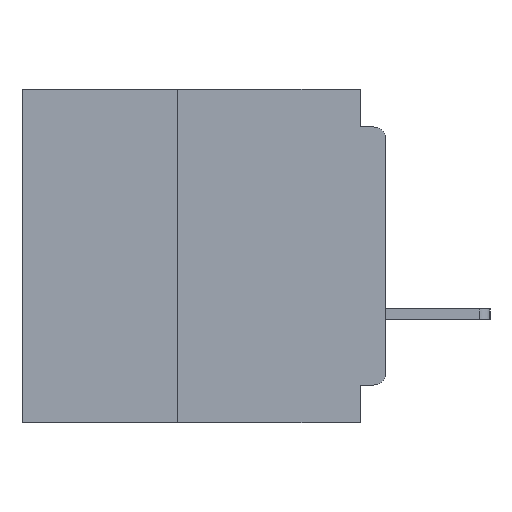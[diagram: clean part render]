
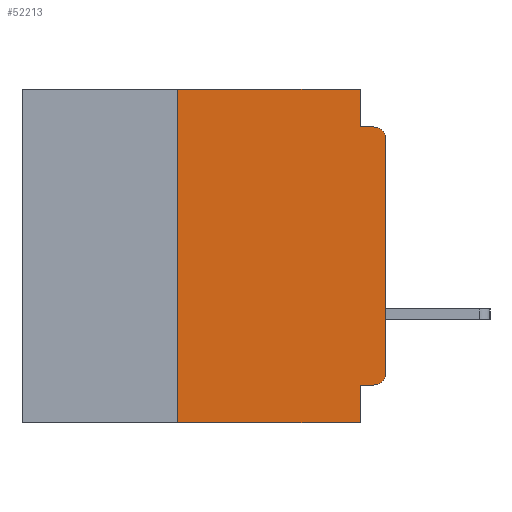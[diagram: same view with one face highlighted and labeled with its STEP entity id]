
A CAD part, left-side view. The second image highlights one B-rep face of the part: STEP entity #52213.
In plain terms, the highlighted planar face has unit normal (-1, 0, 0).
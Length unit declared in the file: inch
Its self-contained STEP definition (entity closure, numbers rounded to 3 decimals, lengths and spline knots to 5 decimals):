
#1529 = CARTESIAN_POINT ( 'NONE',  ( 0., 0., 0. ) ) ;
#2550 = CARTESIAN_POINT ( 'NONE',  ( 0., 0.015, -0.34 ) ) ;
#2847 = CARTESIAN_POINT ( 'NONE',  ( 0., 0.031, 0. ) ) ;
#3229 = CARTESIAN_POINT ( 'NONE',  ( 0., 0.015, -0.355 ) ) ;
#4304 = CARTESIAN_POINT ( 'NONE',  ( 0., 0.437, 0. ) ) ;
#5494 = CARTESIAN_POINT ( 'NONE',  ( 0., 0.25, -0.4 ) ) ;
#7000 = CIRCLE ( 'NONE', #40093, 0.015 ) ;
#7048 = DIRECTION ( 'NONE',  ( 0., 0., -1. ) ) ;
#8974 = CARTESIAN_POINT ( 'NONE',  ( 0., 0.25, -0.4 ) ) ;
#9078 = CARTESIAN_POINT ( 'NONE',  ( 0., 0.031, -0.045 ) ) ;
#9638 = LINE ( 'NONE', #50062, #55705 ) ;
#10190 = EDGE_CURVE ( 'NONE', #34979, #12332, #7000, .T. ) ;
#10256 = ORIENTED_EDGE ( 'NONE', *, *, #56574, .F. ) ;
#10634 = AXIS2_PLACEMENT_3D ( 'NONE', #4304, #17812, #49014 ) ;
#10822 = CARTESIAN_POINT ( 'NONE',  ( 0., 0.031, -0.4 ) ) ;
#11210 = VECTOR ( 'NONE', #27414, 39.37008 ) ;
#11375 = EDGE_CURVE ( 'NONE', #39801, #12332, #9638, .T. ) ;
#11802 = ORIENTED_EDGE ( 'NONE', *, *, #57813, .T. ) ;
#12133 = EDGE_CURVE ( 'NONE', #24165, #34979, #29928, .T. ) ;
#12332 = VERTEX_POINT ( 'NONE', #29952 ) ;
#14647 = ORIENTED_EDGE ( 'NONE', *, *, #12133, .T. ) ;
#15759 = ORIENTED_EDGE ( 'NONE', *, *, #21827, .F. ) ;
#17812 = DIRECTION ( 'NONE',  ( 1., 0., 0. ) ) ;
#18817 = AXIS2_PLACEMENT_3D ( 'NONE', #2550, #33880, #7048 ) ;
#18884 = VERTEX_POINT ( 'NONE', #3229 ) ;
#19562 = DIRECTION ( 'NONE',  ( -1., 0., 0. ) ) ;
#20622 = VERTEX_POINT ( 'NONE', #25210 ) ;
#20630 = VERTEX_POINT ( 'NONE', #2847 ) ;
#20777 = CARTESIAN_POINT ( 'NONE',  ( 0., 0., -0.34 ) ) ;
#21770 = ORIENTED_EDGE ( 'NONE', *, *, #10190, .T. ) ;
#21827 = EDGE_CURVE ( 'NONE', #18884, #37559, #53302, .T. ) ;
#21992 = CARTESIAN_POINT ( 'NONE',  ( 0., 0., -0.355 ) ) ;
#22158 = LINE ( 'NONE', #32784, #29910 ) ;
#22698 = CARTESIAN_POINT ( 'NONE',  ( 0., 0.031, 0. ) ) ;
#22957 = ORIENTED_EDGE ( 'NONE', *, *, #35918, .F. ) ;
#23120 = LINE ( 'NONE', #22698, #11210 ) ;
#24133 = LINE ( 'NONE', #5494, #45021 ) ;
#24165 = VERTEX_POINT ( 'NONE', #20777 ) ;
#24454 = DIRECTION ( 'NONE',  ( 0., 0., -1. ) ) ;
#24993 = ORIENTED_EDGE ( 'NONE', *, *, #26967, .F. ) ;
#25210 = CARTESIAN_POINT ( 'NONE',  ( 0., 0.25, 0. ) ) ;
#26967 = EDGE_CURVE ( 'NONE', #34025, #20622, #24133, .T. ) ;
#27414 = DIRECTION ( 'NONE',  ( 0., 0., -1. ) ) ;
#27470 = FACE_OUTER_BOUND ( 'NONE', #53084, .T. ) ;
#27724 = CIRCLE ( 'NONE', #18817, 0.015 ) ;
#28140 = DIRECTION ( 'NONE',  ( 0., -1., 0. ) ) ;
#29910 = VECTOR ( 'NONE', #37228, 39.37008 ) ;
#29928 = LINE ( 'NONE', #1529, #40310 ) ;
#29952 = CARTESIAN_POINT ( 'NONE',  ( 0., 0.015, -0.045 ) ) ;
#31085 = EDGE_CURVE ( 'NONE', #37559, #42787, #34208, .T. ) ;
#32362 = EDGE_CURVE ( 'NONE', #18884, #24165, #27724, .T. ) ;
#32479 = VECTOR ( 'NONE', #48712, 39.37008 ) ;
#32784 = CARTESIAN_POINT ( 'NONE',  ( 0., 0.437, 0. ) ) ;
#33071 = DIRECTION ( 'NONE',  ( 0., 0., 1. ) ) ;
#33453 = CARTESIAN_POINT ( 'NONE',  ( 0., 0.031, -0.4 ) ) ;
#33880 = DIRECTION ( 'NONE',  ( -1., 0., 0. ) ) ;
#34025 = VERTEX_POINT ( 'NONE', #8974 ) ;
#34208 = LINE ( 'NONE', #33453, #44604 ) ;
#34979 = VERTEX_POINT ( 'NONE', #55684 ) ;
#35918 = EDGE_CURVE ( 'NONE', #20630, #39801, #23120, .T. ) ;
#37228 = DIRECTION ( 'NONE',  ( 0., -1., 0. ) ) ;
#37559 = VERTEX_POINT ( 'NONE', #43934 ) ;
#38675 = ORIENTED_EDGE ( 'NONE', *, *, #32362, .T. ) ;
#39801 = VERTEX_POINT ( 'NONE', #9078 ) ;
#40051 = PLANE ( 'NONE',  #10634 ) ;
#40093 = AXIS2_PLACEMENT_3D ( 'NONE', #46269, #19562, #50775 ) ;
#40310 = VECTOR ( 'NONE', #33071, 39.37008 ) ;
#41211 = DIRECTION ( 'NONE',  ( 0., 0., 1. ) ) ;
#42787 = VERTEX_POINT ( 'NONE', #10822 ) ;
#42933 = LINE ( 'NONE', #54965, #51975 ) ;
#43934 = CARTESIAN_POINT ( 'NONE',  ( 0., 0.031, -0.355 ) ) ;
#44604 = VECTOR ( 'NONE', #24454, 39.37008 ) ;
#45021 = VECTOR ( 'NONE', #41211, 39.37008 ) ;
#46269 = CARTESIAN_POINT ( 'NONE',  ( 0., 0.015, -0.06 ) ) ;
#48712 = DIRECTION ( 'NONE',  ( 0., 1., 0. ) ) ;
#49014 = DIRECTION ( 'NONE',  ( 0., 0., -1. ) ) ;
#50062 = CARTESIAN_POINT ( 'NONE',  ( 0., 0., -0.045 ) ) ;
#50775 = DIRECTION ( 'NONE',  ( 0., 0., -1. ) ) ;
#51975 = VECTOR ( 'NONE', #28140, 39.37008 ) ;
#52213 = ADVANCED_FACE ( 'NONE', ( #27470 ), #40051, .F. ) ;
#53084 = EDGE_LOOP ( 'NONE', ( #14647, #21770, #56055, #22957, #10256, #24993, #11802, #55367, #15759, #38675 ) ) ;
#53302 = LINE ( 'NONE', #21992, #32479 ) ;
#54501 = DIRECTION ( 'NONE',  ( 0., -1., 0. ) ) ;
#54965 = CARTESIAN_POINT ( 'NONE',  ( 0., 0.437, -0.4 ) ) ;
#55367 = ORIENTED_EDGE ( 'NONE', *, *, #31085, .F. ) ;
#55684 = CARTESIAN_POINT ( 'NONE',  ( 0., 0., -0.06 ) ) ;
#55705 = VECTOR ( 'NONE', #54501, 39.37008 ) ;
#56055 = ORIENTED_EDGE ( 'NONE', *, *, #11375, .F. ) ;
#56574 = EDGE_CURVE ( 'NONE', #20622, #20630, #22158, .T. ) ;
#57813 = EDGE_CURVE ( 'NONE', #34025, #42787, #42933, .T. ) ;
